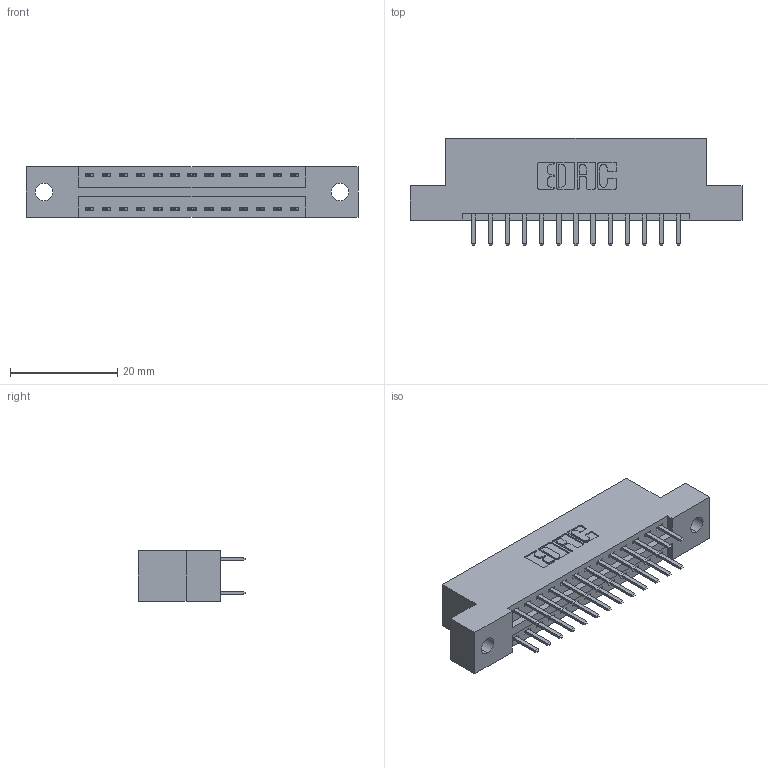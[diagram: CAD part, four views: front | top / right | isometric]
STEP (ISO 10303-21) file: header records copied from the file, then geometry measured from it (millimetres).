
FILE_DESCRIPTION (( 'STEP AP203' ), '1' );
FILE_NAME ('396-026-520-202.STEP', '2019-10-30T04:31:21', ( '' ), ( '' ), 'SwSTEP 2.0', 'SolidWorks 2016', '' );
FILE_SCHEMA (( 'CONFIG_CONTROL_DESIGN' ));
Length unit declared in the file: inch
Products named in the file (3): 396-026-520-202; 346 Part_Flush Mounting Lugs - 0.128 Dia; 345-292-001_345-293-120
Assembly tree (27 placements, depth 2):
  396-026-520-202
    346 Part_Flush Mounting Lugs - 0.128 Dia
    345-292-001_345-293-120  x26
Bounding box: 61.85 x 20.02 x 9.4 mm (x, y, z)
Volume: 5757.7 mm3; surface area: 7162.5 mm2
Topology: 27 solids, 27 shells, 1578 faces, 4567 edges, 2974 vertices
Faces by surface type: plane 1038, cylinder 540
Entity records: 12505 total; most frequent: CARTESIAN_POINT 2112, ORIENTED_EDGE 2034, DIRECTION 1901, EDGE_CURVE 1017, LINE 829, VECTOR 829, VERTEX_POINT 674, AXIS2_PLACEMENT_3D 536
